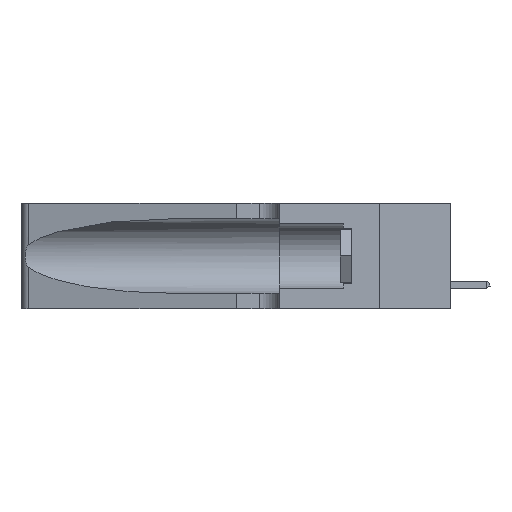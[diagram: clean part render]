
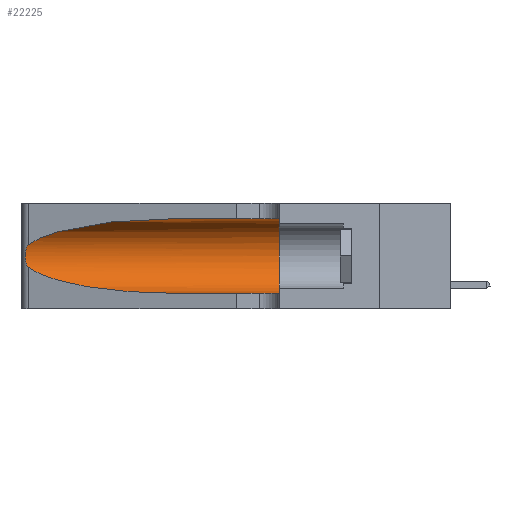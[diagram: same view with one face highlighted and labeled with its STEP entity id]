
A CAD part, left-side view. The second image highlights one B-rep face of the part: STEP entity #22225.
In plain terms, the highlighted cylindrical face has radius 3.308 mm (diameter 6.617 mm), a partial arc.
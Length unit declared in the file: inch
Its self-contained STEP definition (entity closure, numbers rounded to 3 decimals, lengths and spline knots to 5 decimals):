
#238 = AXIS2_PLACEMENT_3D ( 'NONE', #19949, #31879, #35245 ) ;
#483 = VERTEX_POINT ( 'NONE', #39137 ) ;
#566 = VERTEX_POINT ( 'NONE', #36241 ) ;
#1863 = EDGE_CURVE ( 'NONE', #566, #40094, #29162, .T. ) ;
#1888 = DIRECTION ( 'NONE',  ( 0., -1., 0. ) ) ;
#2322 = CARTESIAN_POINT ( 'NONE',  ( 0.25555, 1.22993, 0.14849 ) ) ;
#2822 = CARTESIAN_POINT ( 'NONE',  ( 0.25639, 1.23184, 0.21858 ) ) ;
#2996 = CARTESIAN_POINT ( 'NONE',  ( 0.26075, 1.23896, 0.19203 ) ) ;
#3650 = CARTESIAN_POINT ( 'NONE',  ( 0.1305, 0.35, 0.05475 ) ) ;
#4970 = VERTEX_POINT ( 'NONE', #3650 ) ;
#7224 = ORIENTED_EDGE ( 'NONE', *, *, #46911, .T. ) ;
#7845 = VERTEX_POINT ( 'NONE', #13783 ) ;
#9831 = CARTESIAN_POINT ( 'NONE',  ( 0.25789, 1.23486, 0.15765 ) ) ;
#11479 = CARTESIAN_POINT ( 'NONE',  ( 0.1305, 0.72297, 0.05475 ) ) ;
#12344 = CARTESIAN_POINT ( 'NONE',  ( 0.1305, 1.61858, 0.31525 ) ) ;
#12510 = EDGE_CURVE ( 'NONE', #15566, #4970, #33290, .T. ) ;
#12695 = VECTOR ( 'NONE', #1888, 39.37008 ) ;
#12898 = ORIENTED_EDGE ( 'NONE', *, *, #1863, .F. ) ;
#13060 = FACE_OUTER_BOUND ( 'NONE', #46818, .T. ) ;
#13226 =( BOUNDED_CURVE ( )  B_SPLINE_CURVE ( 3, ( #48227, #43649, #17042, #36072 ),
 .UNSPECIFIED., .F., .F. ) 
 B_SPLINE_CURVE_WITH_KNOTS ( ( 4, 4 ),
 ( 3.44316, 4.71239 ),
 .UNSPECIFIED. ) 
 CURVE ( )  GEOMETRIC_REPRESENTATION_ITEM ( )  RATIONAL_B_SPLINE_CURVE ( ( 1., 0.87, 0.87, 1. ) ) 
 REPRESENTATION_ITEM ( '' )  );
#13717 = CARTESIAN_POINT ( 'NONE',  ( 0.1305, 0.72297, 0.31525 ) ) ;
#13783 = CARTESIAN_POINT ( 'NONE',  ( 0.25487, 1.22718, 0.14631 ) ) ;
#13879 = CARTESIAN_POINT ( 'NONE',  ( 0.1305, 0.35, 0.185 ) ) ;
#15441 = EDGE_CURVE ( 'NONE', #7845, #15566, #13226, .T. ) ;
#15566 = VERTEX_POINT ( 'NONE', #11479 ) ;
#15846 = VECTOR ( 'NONE', #16396, 39.37008 ) ;
#16396 = DIRECTION ( 'NONE',  ( 0., -1., 0. ) ) ;
#17042 = CARTESIAN_POINT ( 'NONE',  ( 0.18966, 0.96281, 0.05475 ) ) ;
#17314 = ORIENTED_EDGE ( 'NONE', *, *, #38490, .T. ) ;
#18625 = ORIENTED_EDGE ( 'NONE', *, *, #15441, .T. ) ;
#18960 = CARTESIAN_POINT ( 'NONE',  ( 0.25487, 1.22718, 0.14631 ) ) ;
#19949 = CARTESIAN_POINT ( 'NONE',  ( 0.1305, 1.61858, 0.185 ) ) ;
#20977 = B_SPLINE_CURVE_WITH_KNOTS ( 'NONE', 3,
 ( #21708, #25557, #2822, #33612, #26029, #44578, #2996, #29920, #25345, #48441, #9831, #40694, #2322, #18960 ),
 .UNSPECIFIED., .F., .F.,
 ( 4, 2, 2, 2, 2, 2, 4 ),
 ( 0., 0.00027, 0.00053, 0.00107, 0.0016, 0.00187, 0.00214 ),
 .UNSPECIFIED. ) ;
#21319 = CARTESIAN_POINT ( 'NONE',  ( 0.18966, 0.96281, 0.31525 ) ) ;
#21708 = CARTESIAN_POINT ( 'NONE',  ( 0.25487, 1.22718, 0.22369 ) ) ;
#21976 = DIRECTION ( 'NONE',  ( 0., 0., 1. ) ) ;
#22225 = ADVANCED_FACE ( 'NONE', ( #13060 ), #46795, .F. ) ;
#22243 = ORIENTED_EDGE ( 'NONE', *, *, #12510, .T. ) ;
#24696 = EDGE_CURVE ( 'NONE', #40094, #4970, #27223, .T. ) ;
#25345 = CARTESIAN_POINT ( 'NONE',  ( 0.26017, 1.23833, 0.17102 ) ) ;
#25557 = CARTESIAN_POINT ( 'NONE',  ( 0.25555, 1.22994, 0.2215 ) ) ;
#26029 = CARTESIAN_POINT ( 'NONE',  ( 0.25854, 1.2359, 0.20912 ) ) ;
#27223 = CIRCLE ( 'NONE', #45199, 0.13025 ) ;
#28315 = CARTESIAN_POINT ( 'NONE',  ( 0.1305, 0.35, 0.31525 ) ) ;
#28976 =( BOUNDED_CURVE ( )  B_SPLINE_CURVE ( 3, ( #13717, #21319, #29069, #44404 ),
 .UNSPECIFIED., .F., .T. ) 
 B_SPLINE_CURVE_WITH_KNOTS ( ( 4, 4 ),
 ( 1.5708, 2.84003 ),
 .UNSPECIFIED. ) 
 CURVE ( )  GEOMETRIC_REPRESENTATION_ITEM ( )  RATIONAL_B_SPLINE_CURVE ( ( 1., 0.87, 0.87, 1. ) ) 
 REPRESENTATION_ITEM ( '' )  );
#29069 = CARTESIAN_POINT ( 'NONE',  ( 0.2373, 1.15595, 0.28018 ) ) ;
#29162 = LINE ( 'NONE', #12344, #15846 ) ;
#29218 = DIRECTION ( 'NONE',  ( 0., 1., 0. ) ) ;
#29920 = CARTESIAN_POINT ( 'NONE',  ( 0.26075, 1.23896, 0.178 ) ) ;
#31314 = CARTESIAN_POINT ( 'NONE',  ( 0.1305, 1.61858, 0.05475 ) ) ;
#31879 = DIRECTION ( 'NONE',  ( 0., -1., 0. ) ) ;
#33290 = LINE ( 'NONE', #31314, #12695 ) ;
#33612 = CARTESIAN_POINT ( 'NONE',  ( 0.25787, 1.23484, 0.2124 ) ) ;
#35245 = DIRECTION ( 'NONE',  ( 0., 0., -1. ) ) ;
#36072 = CARTESIAN_POINT ( 'NONE',  ( 0.1305, 0.72297, 0.05475 ) ) ;
#36241 = CARTESIAN_POINT ( 'NONE',  ( 0.1305, 0.72297, 0.31525 ) ) ;
#38490 = EDGE_CURVE ( 'NONE', #483, #7845, #20977, .T. ) ;
#39137 = CARTESIAN_POINT ( 'NONE',  ( 0.25487, 1.22718, 0.22369 ) ) ;
#40094 = VERTEX_POINT ( 'NONE', #28315 ) ;
#40694 = CARTESIAN_POINT ( 'NONE',  ( 0.25639, 1.23186, 0.15144 ) ) ;
#43649 = CARTESIAN_POINT ( 'NONE',  ( 0.2373, 1.15595, 0.08982 ) ) ;
#44404 = CARTESIAN_POINT ( 'NONE',  ( 0.25487, 1.22718, 0.22369 ) ) ;
#44566 = ORIENTED_EDGE ( 'NONE', *, *, #24696, .F. ) ;
#44578 = CARTESIAN_POINT ( 'NONE',  ( 0.26018, 1.23835, 0.19895 ) ) ;
#45199 = AXIS2_PLACEMENT_3D ( 'NONE', #13879, #29218, #21976 ) ;
#46795 = CYLINDRICAL_SURFACE ( 'NONE', #238, 0.13025 ) ;
#46818 = EDGE_LOOP ( 'NONE', ( #7224, #17314, #18625, #22243, #44566, #12898 ) ) ;
#46911 = EDGE_CURVE ( 'NONE', #566, #483, #28976, .T. ) ;
#48227 = CARTESIAN_POINT ( 'NONE',  ( 0.25487, 1.22718, 0.14631 ) ) ;
#48441 = CARTESIAN_POINT ( 'NONE',  ( 0.25856, 1.23593, 0.16098 ) ) ;
